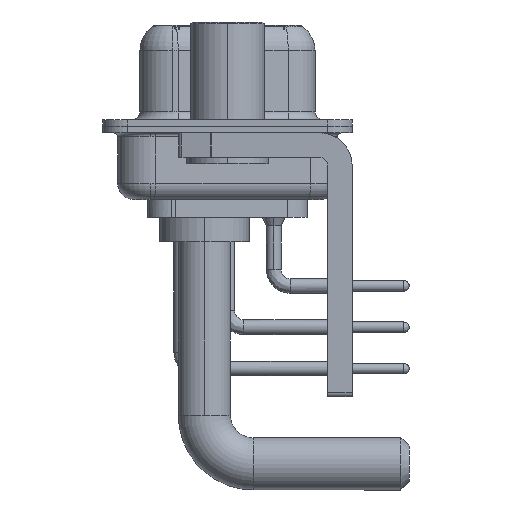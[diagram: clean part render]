
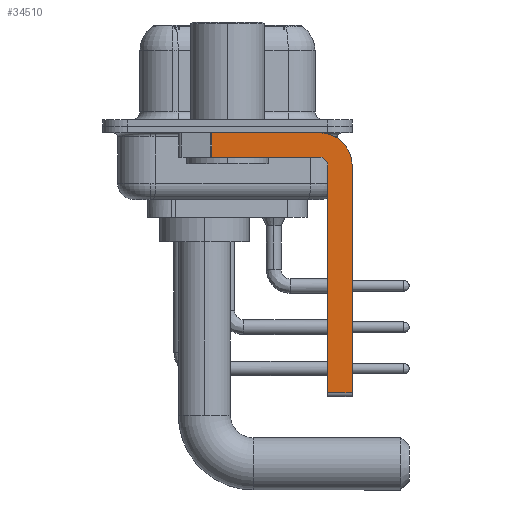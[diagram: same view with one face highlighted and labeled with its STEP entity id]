
A CAD part, left-side view. The second image highlights one B-rep face of the part: STEP entity #34510.
In plain terms, the highlighted planar face has unit normal (-1, 0, 0).
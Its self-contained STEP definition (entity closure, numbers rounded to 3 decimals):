
#1543 = VERTEX_POINT ( 'NONE', #11518 ) ;
#1764 = VECTOR ( 'NONE', #14351, 1000. ) ;
#1958 = VERTEX_POINT ( 'NONE', #33637 ) ;
#2122 = CIRCLE ( 'NONE', #35125, 0.5 ) ;
#3694 = ORIENTED_EDGE ( 'NONE', *, *, #33394, .F. ) ;
#4072 = DIRECTION ( 'NONE',  ( 0., 0., 1. ) ) ;
#5136 = DIRECTION ( 'NONE',  ( 0., 0., -1. ) ) ;
#5242 = CARTESIAN_POINT ( 'NONE',  ( -2.9, -5.65, -2.4 ) ) ;
#6499 = ORIENTED_EDGE ( 'NONE', *, *, #22560, .T. ) ;
#6679 = FACE_OUTER_BOUND ( 'NONE', #24457, .T. ) ;
#6735 = ORIENTED_EDGE ( 'NONE', *, *, #33577, .F. ) ;
#6778 = EDGE_CURVE ( 'NONE', #10294, #29856, #20067, .T. ) ;
#7002 = DIRECTION ( 'NONE',  ( -1., 0., 0. ) ) ;
#9012 = ORIENTED_EDGE ( 'NONE', *, *, #34662, .F. ) ;
#9275 = CARTESIAN_POINT ( 'NONE',  ( -2.9, -5.65, -2.4 ) ) ;
#10156 = LINE ( 'NONE', #32837, #28298 ) ;
#10294 = VERTEX_POINT ( 'NONE', #13575 ) ;
#11518 = CARTESIAN_POINT ( 'NONE',  ( -2.9, -6.15, -16.35 ) ) ;
#11818 = ORIENTED_EDGE ( 'NONE', *, *, #17016, .F. ) ;
#12051 = DIRECTION ( 'NONE',  ( 1., 0., 0. ) ) ;
#12138 = CARTESIAN_POINT ( 'NONE',  ( -2.9, -6.15, -16.6 ) ) ;
#12438 = ORIENTED_EDGE ( 'NONE', *, *, #29250, .T. ) ;
#13046 = CARTESIAN_POINT ( 'NONE',  ( -2.9, -6.15, -2.4 ) ) ;
#13141 = DIRECTION ( 'NONE',  ( 0., -1., 0. ) ) ;
#13575 = CARTESIAN_POINT ( 'NONE',  ( -2.9, -5.65, -1.9 ) ) ;
#13630 = CARTESIAN_POINT ( 'NONE',  ( -2.9, 0.978, -1.9 ) ) ;
#13642 = DIRECTION ( 'NONE',  ( 0., 0., -1. ) ) ;
#14351 = DIRECTION ( 'NONE',  ( 0., 1., 0. ) ) ;
#14629 = VERTEX_POINT ( 'NONE', #25041 ) ;
#15678 = CIRCLE ( 'NONE', #16279, 2. ) ;
#16090 = DIRECTION ( 'NONE',  ( 0., -1., 0. ) ) ;
#16279 = AXIS2_PLACEMENT_3D ( 'NONE', #5242, #33290, #30534 ) ;
#16952 = VERTEX_POINT ( 'NONE', #20286 ) ;
#17016 = EDGE_CURVE ( 'NONE', #23703, #10294, #2122, .T. ) ;
#17712 = EDGE_CURVE ( 'NONE', #16952, #14629, #15678, .T. ) ;
#17817 = ORIENTED_EDGE ( 'NONE', *, *, #17712, .F. ) ;
#18492 = LINE ( 'NONE', #29596, #30075 ) ;
#19140 = LINE ( 'NONE', #30429, #26522 ) ;
#20067 = LINE ( 'NONE', #30969, #1764 ) ;
#20286 = CARTESIAN_POINT ( 'NONE',  ( -2.9, -5.65, -0.4 ) ) ;
#20329 = DIRECTION ( 'NONE',  ( 0., 0., -1. ) ) ;
#22560 = EDGE_CURVE ( 'NONE', #1958, #29856, #19140, .T. ) ;
#22775 = AXIS2_PLACEMENT_3D ( 'NONE', #9275, #12051, #20329 ) ;
#22822 = VERTEX_POINT ( 'NONE', #32433 ) ;
#23451 = CARTESIAN_POINT ( 'NONE',  ( -2.9, -5.65, -2.4 ) ) ;
#23703 = VERTEX_POINT ( 'NONE', #13046 ) ;
#24457 = EDGE_LOOP ( 'NONE', ( #9012, #6499, #35480, #11818, #6735, #12438, #3694, #17817 ) ) ;
#25041 = CARTESIAN_POINT ( 'NONE',  ( -2.9, -7.65, -2.4 ) ) ;
#25345 = VECTOR ( 'NONE', #26546, 1000. ) ;
#26522 = VECTOR ( 'NONE', #5136, 1000. ) ;
#26546 = DIRECTION ( 'NONE',  ( 0., 0., 1. ) ) ;
#26729 = VECTOR ( 'NONE', #13141, 1000. ) ;
#26981 = LINE ( 'NONE', #27178, #26729 ) ;
#27178 = CARTESIAN_POINT ( 'NONE',  ( -2.9, -5.65, -16.35 ) ) ;
#28298 = VECTOR ( 'NONE', #13642, 1000. ) ;
#29250 = EDGE_CURVE ( 'NONE', #1543, #22822, #26981, .T. ) ;
#29596 = CARTESIAN_POINT ( 'NONE',  ( -2.9, 3., -0.4 ) ) ;
#29856 = VERTEX_POINT ( 'NONE', #13630 ) ;
#30075 = VECTOR ( 'NONE', #16090, 1000. ) ;
#30429 = CARTESIAN_POINT ( 'NONE',  ( -2.9, 0.978, -1.9 ) ) ;
#30534 = DIRECTION ( 'NONE',  ( 0., 0., -1. ) ) ;
#30969 = CARTESIAN_POINT ( 'NONE',  ( -2.9, -5.65, -1.9 ) ) ;
#31513 = LINE ( 'NONE', #12138, #25345 ) ;
#31974 = PLANE ( 'NONE',  #22775 ) ;
#32433 = CARTESIAN_POINT ( 'NONE',  ( -2.9, -7.65, -16.35 ) ) ;
#32837 = CARTESIAN_POINT ( 'NONE',  ( -2.9, -7.65, -2.4 ) ) ;
#33290 = DIRECTION ( 'NONE',  ( 1., 0., 0. ) ) ;
#33394 = EDGE_CURVE ( 'NONE', #14629, #22822, #10156, .T. ) ;
#33577 = EDGE_CURVE ( 'NONE', #1543, #23703, #31513, .T. ) ;
#33637 = CARTESIAN_POINT ( 'NONE',  ( -2.9, 0.978, -0.4 ) ) ;
#34510 = ADVANCED_FACE ( 'NONE', ( #6679 ), #31974, .F. ) ;
#34662 = EDGE_CURVE ( 'NONE', #1958, #16952, #18492, .T. ) ;
#35125 = AXIS2_PLACEMENT_3D ( 'NONE', #23451, #7002, #4072 ) ;
#35480 = ORIENTED_EDGE ( 'NONE', *, *, #6778, .F. ) ;
